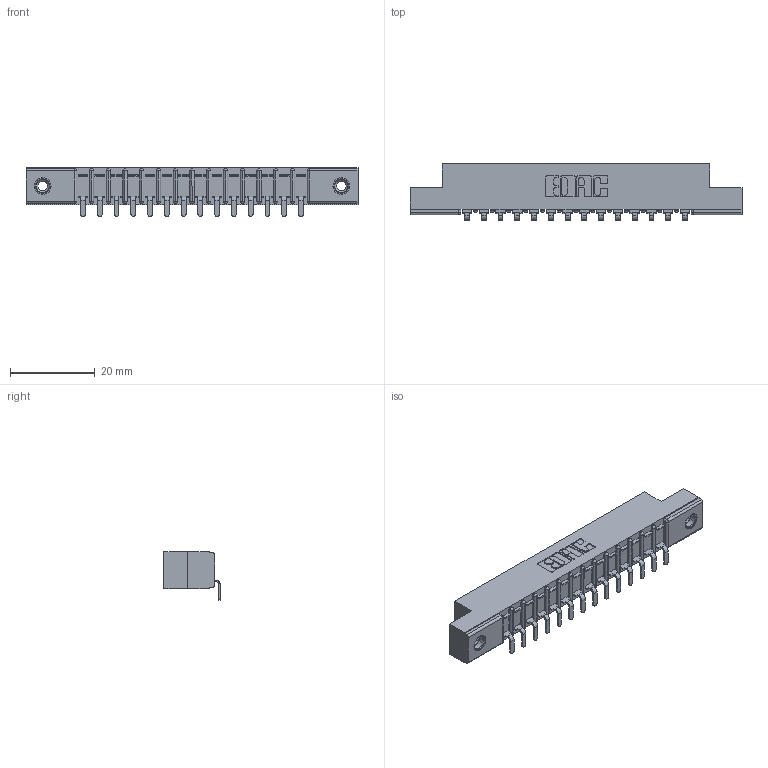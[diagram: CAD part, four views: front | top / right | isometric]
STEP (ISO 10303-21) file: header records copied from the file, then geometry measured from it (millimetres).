
FILE_DESCRIPTION (( 'STEP AP203' ), '1' );
FILE_NAME ('307-014-553-108.STEP', '2018-08-03T00:56:10', ( '' ), ( '' ), 'SwSTEP 2.0', 'SolidWorks 2016', '' );
FILE_SCHEMA (( 'CONFIG_CONTROL_DESIGN' ));
Length unit declared in the file: inch
Products named in the file (4): 307-290-002_553; 345-250-001_345-250-003-102; 307-014-553-108; 307 Part_.156 Dia Mounting Holes
Assembly tree (17 placements, depth 2):
  307-014-553-108
    307 Part_.156 Dia Mounting Holes
    307-290-002_553  x14
    345-250-001_345-250-003-102  x2
Bounding box: 78.49 x 13.32 x 11.51 mm (x, y, z)
Volume: 5170.7 mm3; surface area: 8982.8 mm2
Topology: 17 solids, 17 shells, 1285 faces, 3875 edges, 2534 vertices
Faces by surface type: plane 760, cylinder 479, sphere 30, cone 12, torus 4
Entity records: 17493 total; most frequent: CARTESIAN_POINT 2927, ORIENTED_EDGE 2910, DIRECTION 2867, EDGE_CURVE 1455, LINE 1099, VECTOR 1099, VERTEX_POINT 944, AXIS2_PLACEMENT_3D 884
